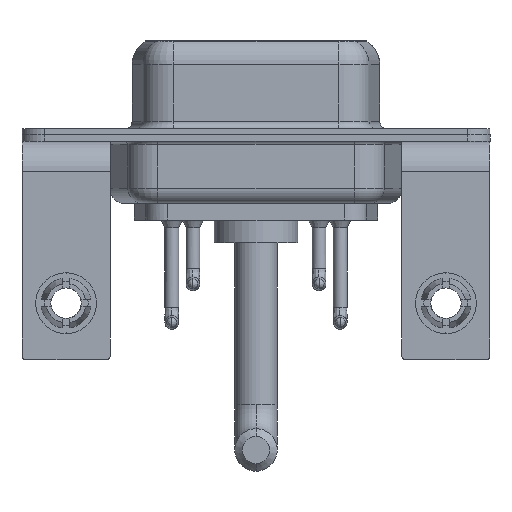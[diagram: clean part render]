
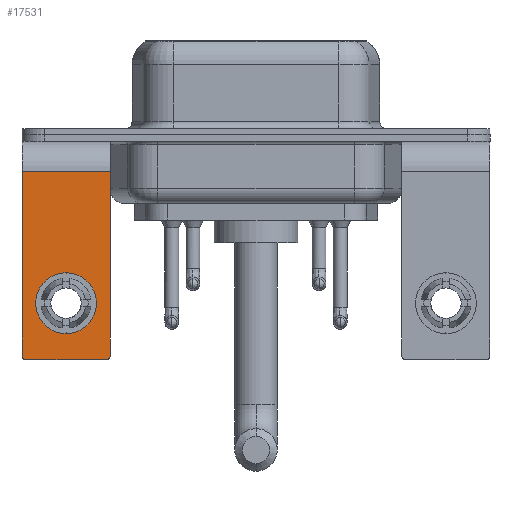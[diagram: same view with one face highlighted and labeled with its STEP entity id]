
A CAD part, front view. The second image highlights one B-rep face of the part: STEP entity #17531.
In plain terms, the highlighted planar face has unit normal (0, -1, 0).
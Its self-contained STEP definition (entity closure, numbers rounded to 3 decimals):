
#9 = VERTEX_POINT ( 'NONE', #13720 ) ;
#69 = DIRECTION ( 'NONE',  ( -1., 0., 0. ) ) ;
#250 = CARTESIAN_POINT ( 'NONE',  ( 2.9, -6.25, -14.8 ) ) ;
#287 = CARTESIAN_POINT ( 'NONE',  ( 0., -6.25, -13.07 ) ) ;
#734 = DIRECTION ( 'NONE',  ( 0., 0., -1. ) ) ;
#809 = AXIS2_PLACEMENT_3D ( 'NONE', #5936, #7541, #17484 ) ;
#862 = ORIENTED_EDGE ( 'NONE', *, *, #17301, .T. ) ;
#1307 = EDGE_CURVE ( 'NONE', #7742, #14535, #7004, .T. ) ;
#1425 = DIRECTION ( 'NONE',  ( 0., 0., -1. ) ) ;
#1509 = DIRECTION ( 'NONE',  ( 0., -1., 0. ) ) ;
#1515 = CARTESIAN_POINT ( 'NONE',  ( 2.9, -6.25, -2.4 ) ) ;
#1939 = CARTESIAN_POINT ( 'NONE',  ( 2.9, -6.25, -2.4 ) ) ;
#1947 = EDGE_CURVE ( 'NONE', #17228, #14535, #13817, .T. ) ;
#2780 = VERTEX_POINT ( 'NONE', #287 ) ;
#3186 = CARTESIAN_POINT ( 'NONE',  ( -2.65, -6.25, -14.8 ) ) ;
#3363 = ORIENTED_EDGE ( 'NONE', *, *, #9242, .T. ) ;
#3560 = CARTESIAN_POINT ( 'NONE',  ( 2.9, -6.25, -2.4 ) ) ;
#3638 = DIRECTION ( 'NONE',  ( 0., 1., 0. ) ) ;
#3897 = EDGE_CURVE ( 'NONE', #7742, #16469, #6572, .T. ) ;
#4131 = EDGE_LOOP ( 'NONE', ( #862, #18303 ) ) ;
#4404 = VERTEX_POINT ( 'NONE', #13950 ) ;
#4563 = CIRCLE ( 'NONE', #11811, 2. ) ;
#5639 = CARTESIAN_POINT ( 'NONE',  ( 0., -6.25, -11.07 ) ) ;
#5936 = CARTESIAN_POINT ( 'NONE',  ( 2.65, -6.25, -14.55 ) ) ;
#6092 = DIRECTION ( 'NONE',  ( 0., 0., 1. ) ) ;
#6375 = FACE_BOUND ( 'NONE', #4131, .T. ) ;
#6386 = DIRECTION ( 'NONE',  ( -1., 0., 0. ) ) ;
#6572 = LINE ( 'NONE', #3560, #14434 ) ;
#6638 = ORIENTED_EDGE ( 'NONE', *, *, #15999, .T. ) ;
#6687 = CARTESIAN_POINT ( 'NONE',  ( -2.9, -6.25, -2.4 ) ) ;
#7004 = LINE ( 'NONE', #1515, #11960 ) ;
#7272 = DIRECTION ( 'NONE',  ( 0., 0., 1. ) ) ;
#7541 = DIRECTION ( 'NONE',  ( 0., -1., 0. ) ) ;
#7567 = EDGE_CURVE ( 'NONE', #9, #2780, #4563, .T. ) ;
#7691 = VECTOR ( 'NONE', #69, 1000. ) ;
#7742 = VERTEX_POINT ( 'NONE', #1939 ) ;
#8276 = AXIS2_PLACEMENT_3D ( 'NONE', #5639, #17176, #12745 ) ;
#8409 = VERTEX_POINT ( 'NONE', #3186 ) ;
#8517 = ORIENTED_EDGE ( 'NONE', *, *, #1947, .T. ) ;
#8859 = ORIENTED_EDGE ( 'NONE', *, *, #3897, .T. ) ;
#8873 = ORIENTED_EDGE ( 'NONE', *, *, #9513, .F. ) ;
#9218 = FACE_OUTER_BOUND ( 'NONE', #15907, .T. ) ;
#9242 = EDGE_CURVE ( 'NONE', #16469, #4404, #13713, .T. ) ;
#9513 = EDGE_CURVE ( 'NONE', #17228, #8409, #13220, .T. ) ;
#10933 = CIRCLE ( 'NONE', #12459, 0.25 ) ;
#11536 = CARTESIAN_POINT ( 'NONE',  ( 2.9, -6.25, -14.55 ) ) ;
#11718 = CARTESIAN_POINT ( 'NONE',  ( -2.65, -6.25, -14.55 ) ) ;
#11811 = AXIS2_PLACEMENT_3D ( 'NONE', #12928, #17356, #6092 ) ;
#11960 = VECTOR ( 'NONE', #1425, 1000. ) ;
#12459 = AXIS2_PLACEMENT_3D ( 'NONE', #11718, #1509, #7272 ) ;
#12745 = DIRECTION ( 'NONE',  ( 0., 0., 1. ) ) ;
#12928 = CARTESIAN_POINT ( 'NONE',  ( 0., -6.25, -11.07 ) ) ;
#13220 = LINE ( 'NONE', #250, #7691 ) ;
#13713 = LINE ( 'NONE', #6687, #17686 ) ;
#13720 = CARTESIAN_POINT ( 'NONE',  ( 0., -6.25, -9.07 ) ) ;
#13817 = CIRCLE ( 'NONE', #809, 0.25 ) ;
#13950 = CARTESIAN_POINT ( 'NONE',  ( -2.9, -6.25, -14.55 ) ) ;
#14037 = AXIS2_PLACEMENT_3D ( 'NONE', #15181, #3638, #14909 ) ;
#14434 = VECTOR ( 'NONE', #6386, 1000. ) ;
#14535 = VERTEX_POINT ( 'NONE', #11536 ) ;
#14909 = DIRECTION ( 'NONE',  ( 0., 0., 1. ) ) ;
#15181 = CARTESIAN_POINT ( 'NONE',  ( 2.9, -6.25, -2.4 ) ) ;
#15478 = CARTESIAN_POINT ( 'NONE',  ( 2.65, -6.25, -14.8 ) ) ;
#15907 = EDGE_LOOP ( 'NONE', ( #3363, #6638, #8873, #8517, #15952, #8859 ) ) ;
#15952 = ORIENTED_EDGE ( 'NONE', *, *, #1307, .F. ) ;
#15999 = EDGE_CURVE ( 'NONE', #4404, #8409, #10933, .T. ) ;
#16139 = CARTESIAN_POINT ( 'NONE',  ( -2.9, -6.25, -2.4 ) ) ;
#16469 = VERTEX_POINT ( 'NONE', #16139 ) ;
#17049 = CIRCLE ( 'NONE', #8276, 2. ) ;
#17176 = DIRECTION ( 'NONE',  ( 0., 1., 0. ) ) ;
#17228 = VERTEX_POINT ( 'NONE', #15478 ) ;
#17301 = EDGE_CURVE ( 'NONE', #2780, #9, #17049, .T. ) ;
#17356 = DIRECTION ( 'NONE',  ( 0., 1., 0. ) ) ;
#17484 = DIRECTION ( 'NONE',  ( 0., 0., 1. ) ) ;
#17531 = ADVANCED_FACE ( 'NONE', ( #6375, #9218 ), #17831, .F. ) ;
#17686 = VECTOR ( 'NONE', #734, 1000. ) ;
#17831 = PLANE ( 'NONE',  #14037 ) ;
#18303 = ORIENTED_EDGE ( 'NONE', *, *, #7567, .T. ) ;
